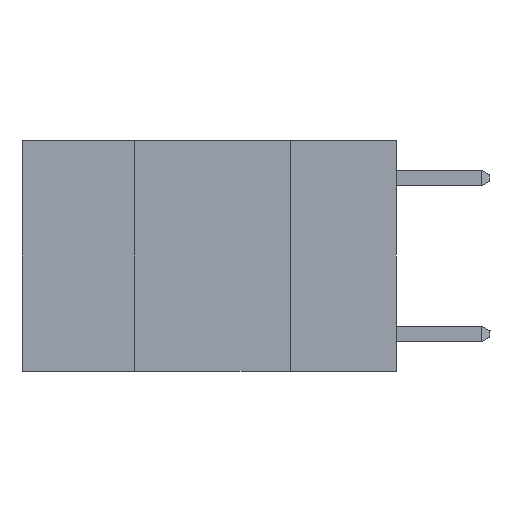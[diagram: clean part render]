
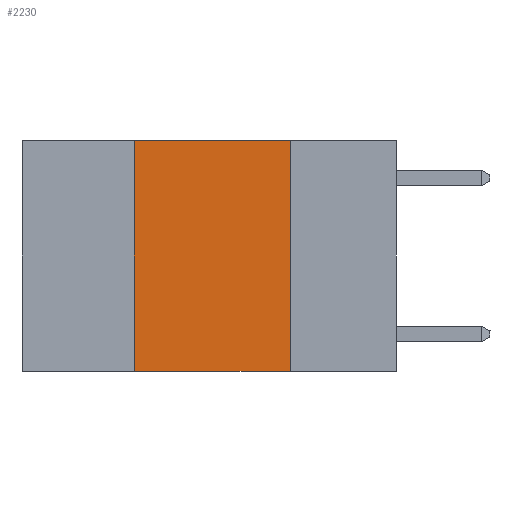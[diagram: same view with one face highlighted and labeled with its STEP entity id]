
A CAD part, left-side view. The second image highlights one B-rep face of the part: STEP entity #2230.
In plain terms, the highlighted planar face has unit normal (-1, 0, 0).
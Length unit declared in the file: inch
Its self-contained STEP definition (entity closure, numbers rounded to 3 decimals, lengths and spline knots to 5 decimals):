
#63 = PLANE ( 'NONE',  #10473 ) ;
#161 = ORIENTED_EDGE ( 'NONE', *, *, #5401, .T. ) ;
#387 = CARTESIAN_POINT ( 'NONE',  ( 0., 0.42, 0. ) ) ;
#497 = DIRECTION ( 'NONE',  ( 0., -1., 0. ) ) ;
#595 = ORIENTED_EDGE ( 'NONE', *, *, #10644, .F. ) ;
#1014 = CARTESIAN_POINT ( 'NONE',  ( 0., 0.42, -0.37 ) ) ;
#1049 = DIRECTION ( 'NONE',  ( 0., 0., -1. ) ) ;
#1187 = DIRECTION ( 'NONE',  ( 0., 0., 1. ) ) ;
#1542 = LINE ( 'NONE', #8379, #7142 ) ;
#2067 = CARTESIAN_POINT ( 'NONE',  ( 0., 0.17, 0. ) ) ;
#2230 = ADVANCED_FACE ( 'NONE', ( #4614 ), #63, .F. ) ;
#2322 = EDGE_CURVE ( 'NONE', #9101, #6571, #11196, .T. ) ;
#3162 = VECTOR ( 'NONE', #5276, 39.37008 ) ;
#3604 = ORIENTED_EDGE ( 'NONE', *, *, #2322, .F. ) ;
#4614 = FACE_OUTER_BOUND ( 'NONE', #8864, .T. ) ;
#5276 = DIRECTION ( 'NONE',  ( 0., 0., -1. ) ) ;
#5401 = EDGE_CURVE ( 'NONE', #9101, #8512, #8882, .T. ) ;
#5798 = LINE ( 'NONE', #8248, #3162 ) ;
#5817 = VERTEX_POINT ( 'NONE', #2067 ) ;
#5907 = VECTOR ( 'NONE', #497, 39.37008 ) ;
#5978 = VECTOR ( 'NONE', #1187, 39.37008 ) ;
#6381 = DIRECTION ( 'NONE',  ( 0., -1., 0. ) ) ;
#6571 = VERTEX_POINT ( 'NONE', #387 ) ;
#7015 = DIRECTION ( 'NONE',  ( 1., 0., 0. ) ) ;
#7142 = VECTOR ( 'NONE', #6381, 39.37008 ) ;
#7152 = CARTESIAN_POINT ( 'NONE',  ( 0., 0.42, 0. ) ) ;
#7498 = ORIENTED_EDGE ( 'NONE', *, *, #8737, .F. ) ;
#7879 = CARTESIAN_POINT ( 'NONE',  ( 0., 0.17, -0.37 ) ) ;
#8248 = CARTESIAN_POINT ( 'NONE',  ( 0., 0.17, 0. ) ) ;
#8379 = CARTESIAN_POINT ( 'NONE',  ( 0., 0.6, 0. ) ) ;
#8512 = VERTEX_POINT ( 'NONE', #7879 ) ;
#8737 = EDGE_CURVE ( 'NONE', #5817, #8512, #5798, .T. ) ;
#8864 = EDGE_LOOP ( 'NONE', ( #7498, #595, #3604, #161 ) ) ;
#8882 = LINE ( 'NONE', #10376, #5907 ) ;
#9101 = VERTEX_POINT ( 'NONE', #1014 ) ;
#9967 = CARTESIAN_POINT ( 'NONE',  ( 0., 0.6, 0. ) ) ;
#10376 = CARTESIAN_POINT ( 'NONE',  ( 0., 0.6, -0.37 ) ) ;
#10473 = AXIS2_PLACEMENT_3D ( 'NONE', #9967, #7015, #1049 ) ;
#10644 = EDGE_CURVE ( 'NONE', #6571, #5817, #1542, .T. ) ;
#11196 = LINE ( 'NONE', #7152, #5978 ) ;
